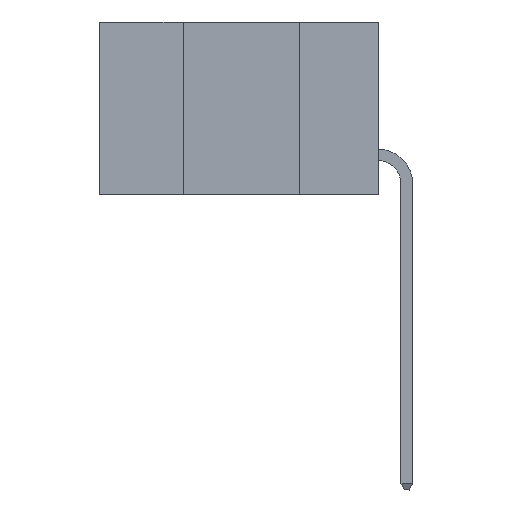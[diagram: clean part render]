
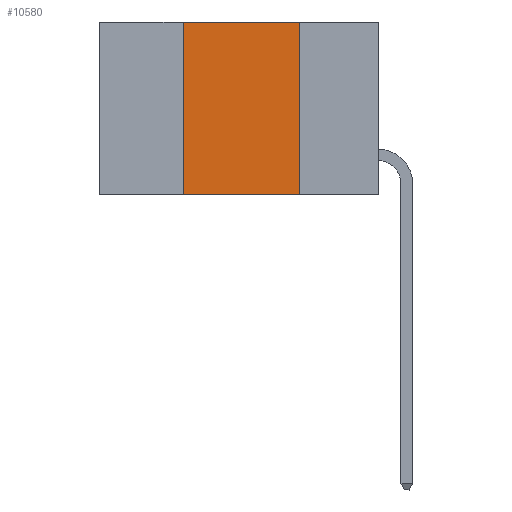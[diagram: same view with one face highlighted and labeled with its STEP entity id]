
A CAD part, left-side view. The second image highlights one B-rep face of the part: STEP entity #10580.
In plain terms, the highlighted planar face has unit normal (-1, 0, 0).
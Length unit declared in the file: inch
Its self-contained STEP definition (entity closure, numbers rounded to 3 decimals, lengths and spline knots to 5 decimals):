
#693 = ORIENTED_EDGE ( 'NONE', *, *, #6201, .F. ) ;
#1086 = CARTESIAN_POINT ( 'NONE',  ( 0., 0.6, -0.37 ) ) ;
#1699 = VERTEX_POINT ( 'NONE', #9283 ) ;
#2145 = CARTESIAN_POINT ( 'NONE',  ( 0., 0.42, -0.37 ) ) ;
#2507 = EDGE_CURVE ( 'NONE', #7822, #1699, #11526, .T. ) ;
#2571 = CARTESIAN_POINT ( 'NONE',  ( 0., 0.42, 0. ) ) ;
#2658 = CARTESIAN_POINT ( 'NONE',  ( 0., 0.17, 0. ) ) ;
#2792 = VECTOR ( 'NONE', #3777, 39.37008 ) ;
#3161 = CARTESIAN_POINT ( 'NONE',  ( 0., 0.17, -0.37 ) ) ;
#3777 = DIRECTION ( 'NONE',  ( 0., 0., 1. ) ) ;
#4241 = LINE ( 'NONE', #2658, #9984 ) ;
#4663 = EDGE_CURVE ( 'NONE', #14794, #7628, #13867, .T. ) ;
#5426 = EDGE_CURVE ( 'NONE', #14794, #7822, #13843, .T. ) ;
#6153 = AXIS2_PLACEMENT_3D ( 'NONE', #6216, #14144, #7411 ) ;
#6201 = EDGE_CURVE ( 'NONE', #1699, #7628, #4241, .T. ) ;
#6216 = CARTESIAN_POINT ( 'NONE',  ( 0., 0.6, 0. ) ) ;
#6398 = EDGE_LOOP ( 'NONE', ( #693, #9951, #7290, #10296 ) ) ;
#7290 = ORIENTED_EDGE ( 'NONE', *, *, #5426, .F. ) ;
#7411 = DIRECTION ( 'NONE',  ( 0., 0., -1. ) ) ;
#7628 = VERTEX_POINT ( 'NONE', #3161 ) ;
#7822 = VERTEX_POINT ( 'NONE', #13689 ) ;
#9212 = DIRECTION ( 'NONE',  ( 0., -1., 0. ) ) ;
#9283 = CARTESIAN_POINT ( 'NONE',  ( 0., 0.17, 0. ) ) ;
#9481 = DIRECTION ( 'NONE',  ( 0., -1., 0. ) ) ;
#9658 = CARTESIAN_POINT ( 'NONE',  ( 0., 0.6, 0. ) ) ;
#9951 = ORIENTED_EDGE ( 'NONE', *, *, #2507, .F. ) ;
#9984 = VECTOR ( 'NONE', #14081, 39.37008 ) ;
#10296 = ORIENTED_EDGE ( 'NONE', *, *, #4663, .T. ) ;
#10580 = ADVANCED_FACE ( 'NONE', ( #12032 ), #13044, .F. ) ;
#11526 = LINE ( 'NONE', #9658, #11910 ) ;
#11910 = VECTOR ( 'NONE', #9481, 39.37008 ) ;
#12032 = FACE_OUTER_BOUND ( 'NONE', #6398, .T. ) ;
#13044 = PLANE ( 'NONE',  #6153 ) ;
#13689 = CARTESIAN_POINT ( 'NONE',  ( 0., 0.42, 0. ) ) ;
#13843 = LINE ( 'NONE', #2571, #2792 ) ;
#13867 = LINE ( 'NONE', #1086, #14225 ) ;
#14081 = DIRECTION ( 'NONE',  ( 0., 0., -1. ) ) ;
#14144 = DIRECTION ( 'NONE',  ( 1., 0., 0. ) ) ;
#14225 = VECTOR ( 'NONE', #9212, 39.37008 ) ;
#14794 = VERTEX_POINT ( 'NONE', #2145 ) ;
